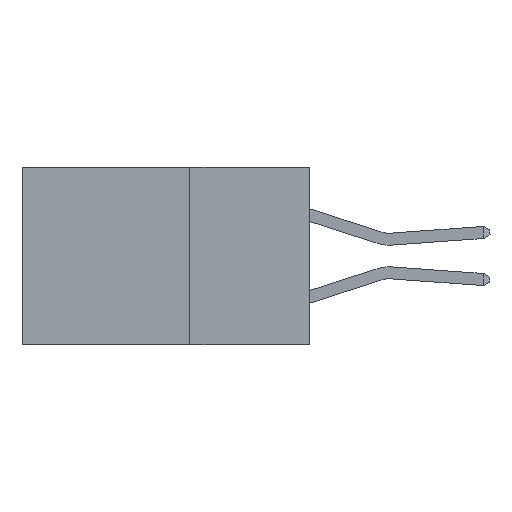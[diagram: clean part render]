
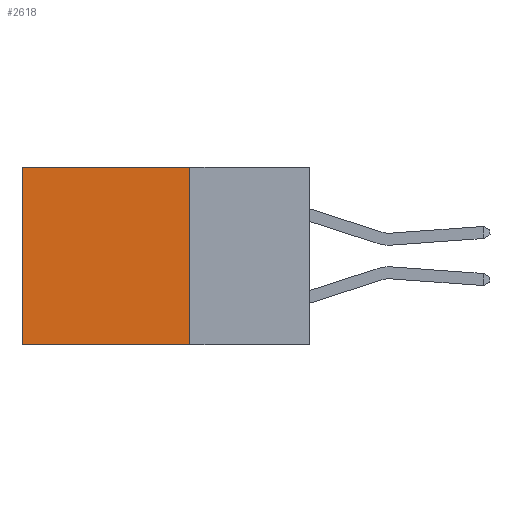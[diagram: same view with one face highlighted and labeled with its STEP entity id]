
A CAD part, left-side view. The second image highlights one B-rep face of the part: STEP entity #2618.
In plain terms, the highlighted planar face has unit normal (-1, 0, 0).
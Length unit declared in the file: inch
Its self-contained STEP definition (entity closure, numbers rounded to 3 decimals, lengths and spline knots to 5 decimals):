
#397 = CARTESIAN_POINT ( 'NONE',  ( 0.298, 0.25, 0. ) ) ;
#1891 = LINE ( 'NONE', #9877, #15764 ) ;
#2578 = ORIENTED_EDGE ( 'NONE', *, *, #21976, .T. ) ;
#2618 = ADVANCED_FACE ( 'NONE', ( #15284 ), #12023, .F. ) ;
#3373 = VECTOR ( 'NONE', #14218, 39.37008 ) ;
#4591 = LINE ( 'NONE', #9497, #3373 ) ;
#5045 = DIRECTION ( 'NONE',  ( 1., 0., 0. ) ) ;
#5071 = DIRECTION ( 'NONE',  ( 0., 0., -1. ) ) ;
#5172 = CARTESIAN_POINT ( 'NONE',  ( 0.298, 0.6, 0. ) ) ;
#5339 = VECTOR ( 'NONE', #11283, 39.37008 ) ;
#6129 = VECTOR ( 'NONE', #14473, 39.37008 ) ;
#6646 = VERTEX_POINT ( 'NONE', #20295 ) ;
#7695 = ORIENTED_EDGE ( 'NONE', *, *, #20816, .F. ) ;
#7972 = DIRECTION ( 'NONE',  ( 0., 0., -1. ) ) ;
#8750 = ORIENTED_EDGE ( 'NONE', *, *, #17676, .F. ) ;
#9497 = CARTESIAN_POINT ( 'NONE',  ( 0.298, 0.25, -0.37 ) ) ;
#9877 = CARTESIAN_POINT ( 'NONE',  ( 0.298, 0.6, 0. ) ) ;
#9955 = VERTEX_POINT ( 'NONE', #15144 ) ;
#11283 = DIRECTION ( 'NONE',  ( 0., 1., 0. ) ) ;
#12023 = PLANE ( 'NONE',  #20012 ) ;
#12623 = CARTESIAN_POINT ( 'NONE',  ( 0.298, 0.25, 0. ) ) ;
#14218 = DIRECTION ( 'NONE',  ( 0., 1., 0. ) ) ;
#14473 = DIRECTION ( 'NONE',  ( 0., 0., -1. ) ) ;
#14522 = EDGE_CURVE ( 'NONE', #14843, #21696, #1891, .T. ) ;
#14843 = VERTEX_POINT ( 'NONE', #5172 ) ;
#15144 = CARTESIAN_POINT ( 'NONE',  ( 0.298, 0.25, -0.37 ) ) ;
#15284 = FACE_OUTER_BOUND ( 'NONE', #18518, .T. ) ;
#15764 = VECTOR ( 'NONE', #7972, 39.37008 ) ;
#16930 = ORIENTED_EDGE ( 'NONE', *, *, #14522, .T. ) ;
#17676 = EDGE_CURVE ( 'NONE', #6646, #9955, #20347, .T. ) ;
#18518 = EDGE_LOOP ( 'NONE', ( #16930, #7695, #8750, #2578 ) ) ;
#18620 = CARTESIAN_POINT ( 'NONE',  ( 0.298, 0.25, 0. ) ) ;
#19673 = CARTESIAN_POINT ( 'NONE',  ( 0.298, 0.6, -0.37 ) ) ;
#20012 = AXIS2_PLACEMENT_3D ( 'NONE', #397, #5045, #5071 ) ;
#20295 = CARTESIAN_POINT ( 'NONE',  ( 0.298, 0.25, 0. ) ) ;
#20347 = LINE ( 'NONE', #12623, #6129 ) ;
#20816 = EDGE_CURVE ( 'NONE', #9955, #21696, #4591, .T. ) ;
#21696 = VERTEX_POINT ( 'NONE', #19673 ) ;
#21976 = EDGE_CURVE ( 'NONE', #6646, #14843, #23843, .T. ) ;
#23843 = LINE ( 'NONE', #18620, #5339 ) ;
